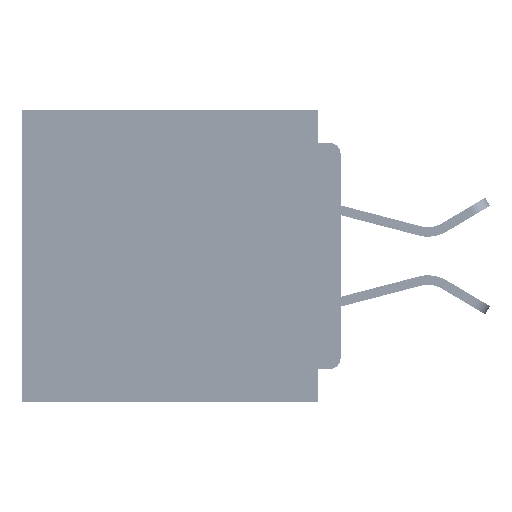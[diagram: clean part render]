
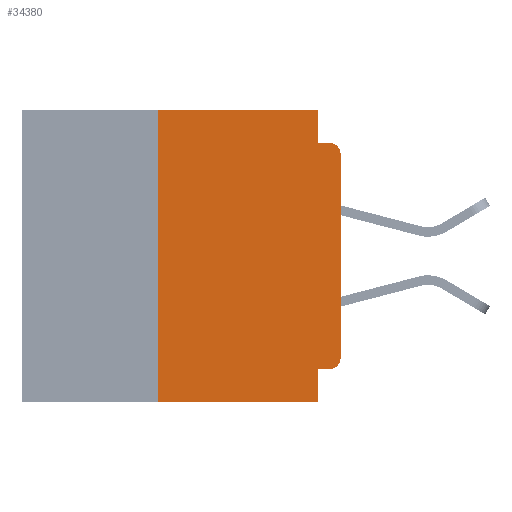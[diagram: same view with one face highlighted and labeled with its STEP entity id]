
A CAD part, left-side view. The second image highlights one B-rep face of the part: STEP entity #34380.
In plain terms, the highlighted planar face has unit normal (-1, 0, 0).
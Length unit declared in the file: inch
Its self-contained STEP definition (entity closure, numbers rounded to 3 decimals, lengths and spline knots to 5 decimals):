
#99 = VECTOR ( 'NONE', #842, 39.37008 ) ;
#659 = VECTOR ( 'NONE', #51162, 39.37008 ) ;
#842 = DIRECTION ( 'NONE',  ( 0., 0., -1. ) ) ;
#1524 = EDGE_CURVE ( 'NONE', #34058, #25634, #24173, .T. ) ;
#1538 = CARTESIAN_POINT ( 'NONE',  ( 0., 0., -0.34 ) ) ;
#2293 = VERTEX_POINT ( 'NONE', #41181 ) ;
#2834 = VECTOR ( 'NONE', #7046, 39.37008 ) ;
#2990 = CARTESIAN_POINT ( 'NONE',  ( 0., 0.031, -0.4 ) ) ;
#5468 = VECTOR ( 'NONE', #60756, 39.37008 ) ;
#6191 = CARTESIAN_POINT ( 'NONE',  ( 0., 0.015, -0.355 ) ) ;
#6379 = CARTESIAN_POINT ( 'NONE',  ( 0., 0.015, -0.34 ) ) ;
#7046 = DIRECTION ( 'NONE',  ( 0., -1., 0. ) ) ;
#7738 = VERTEX_POINT ( 'NONE', #44870 ) ;
#7950 = CARTESIAN_POINT ( 'NONE',  ( 0., 0.015, -0.045 ) ) ;
#8691 = DIRECTION ( 'NONE',  ( 0., 0., -1. ) ) ;
#9320 = EDGE_CURVE ( 'NONE', #7738, #52617, #40028, .T. ) ;
#9327 = AXIS2_PLACEMENT_3D ( 'NONE', #32891, #37742, #8691 ) ;
#9519 = AXIS2_PLACEMENT_3D ( 'NONE', #54440, #25648, #59216 ) ;
#9685 = AXIS2_PLACEMENT_3D ( 'NONE', #6379, #40273, #11241 ) ;
#10809 = DIRECTION ( 'NONE',  ( 0., -1., 0. ) ) ;
#11241 = DIRECTION ( 'NONE',  ( 0., 0., -1. ) ) ;
#11503 = EDGE_CURVE ( 'NONE', #52617, #2293, #13530, .T. ) ;
#11518 = CIRCLE ( 'NONE', #9685, 0.015 ) ;
#13530 = LINE ( 'NONE', #46327, #659 ) ;
#13780 = VECTOR ( 'NONE', #10809, 39.37008 ) ;
#15394 = EDGE_CURVE ( 'NONE', #29434, #55348, #33527, .T. ) ;
#15778 = VECTOR ( 'NONE', #33908, 39.37008 ) ;
#16578 = CARTESIAN_POINT ( 'NONE',  ( 0., 0., -0.045 ) ) ;
#16606 = CARTESIAN_POINT ( 'NONE',  ( 0., 0.25, -0.4 ) ) ;
#16900 = ORIENTED_EDGE ( 'NONE', *, *, #9320, .F. ) ;
#17994 = EDGE_LOOP ( 'NONE', ( #53447, #20706, #44732, #55438, #33008, #16900, #32135, #35148, #19680, #34286 ) ) ;
#18685 = CIRCLE ( 'NONE', #9519, 0.015 ) ;
#19680 = ORIENTED_EDGE ( 'NONE', *, *, #1524, .F. ) ;
#20377 = CARTESIAN_POINT ( 'NONE',  ( 0., 0.437, -0.4 ) ) ;
#20535 = FACE_OUTER_BOUND ( 'NONE', #17994, .T. ) ;
#20706 = ORIENTED_EDGE ( 'NONE', *, *, #41614, .T. ) ;
#21801 = CARTESIAN_POINT ( 'NONE',  ( 0., 0.031, -0.4 ) ) ;
#23041 = EDGE_CURVE ( 'NONE', #2293, #54435, #59716, .T. ) ;
#23720 = VECTOR ( 'NONE', #58821, 39.37008 ) ;
#24173 = LINE ( 'NONE', #54719, #48326 ) ;
#24492 = EDGE_CURVE ( 'NONE', #25634, #38003, #31297, .T. ) ;
#25039 = CARTESIAN_POINT ( 'NONE',  ( 0., 0.031, 0. ) ) ;
#25634 = VERTEX_POINT ( 'NONE', #30950 ) ;
#25648 = DIRECTION ( 'NONE',  ( -1., 0., 0. ) ) ;
#26277 = CARTESIAN_POINT ( 'NONE',  ( 0., 0.25, 0. ) ) ;
#29434 = VERTEX_POINT ( 'NONE', #1538 ) ;
#30107 = CARTESIAN_POINT ( 'NONE',  ( 0., 0., 0. ) ) ;
#30950 = CARTESIAN_POINT ( 'NONE',  ( 0., 0.031, -0.355 ) ) ;
#31297 = LINE ( 'NONE', #2990, #5468 ) ;
#32135 = ORIENTED_EDGE ( 'NONE', *, *, #51992, .T. ) ;
#32764 = VERTEX_POINT ( 'NONE', #7950 ) ;
#32891 = CARTESIAN_POINT ( 'NONE',  ( 0., 0.437, 0. ) ) ;
#33008 = ORIENTED_EDGE ( 'NONE', *, *, #11503, .F. ) ;
#33527 = LINE ( 'NONE', #30107, #23720 ) ;
#33690 = EDGE_CURVE ( 'NONE', #34058, #29434, #11518, .T. ) ;
#33908 = DIRECTION ( 'NONE',  ( 0., 0., 1. ) ) ;
#34058 = VERTEX_POINT ( 'NONE', #6191 ) ;
#34286 = ORIENTED_EDGE ( 'NONE', *, *, #33690, .T. ) ;
#34380 = ADVANCED_FACE ( 'NONE', ( #20535 ), #61557, .F. ) ;
#35148 = ORIENTED_EDGE ( 'NONE', *, *, #24492, .F. ) ;
#37742 = DIRECTION ( 'NONE',  ( 1., 0., 0. ) ) ;
#38003 = VERTEX_POINT ( 'NONE', #21801 ) ;
#40028 = LINE ( 'NONE', #16606, #15778 ) ;
#40273 = DIRECTION ( 'NONE',  ( -1., 0., 0. ) ) ;
#41181 = CARTESIAN_POINT ( 'NONE',  ( 0., 0.031, 0. ) ) ;
#41521 = LINE ( 'NONE', #16578, #2834 ) ;
#41614 = EDGE_CURVE ( 'NONE', #55348, #32764, #18685, .T. ) ;
#42900 = CARTESIAN_POINT ( 'NONE',  ( 0., 0.031, -0.045 ) ) ;
#44732 = ORIENTED_EDGE ( 'NONE', *, *, #59800, .F. ) ;
#44870 = CARTESIAN_POINT ( 'NONE',  ( 0., 0.25, -0.4 ) ) ;
#46327 = CARTESIAN_POINT ( 'NONE',  ( 0., 0.437, 0. ) ) ;
#48326 = VECTOR ( 'NONE', #55194, 39.37008 ) ;
#51162 = DIRECTION ( 'NONE',  ( 0., -1., 0. ) ) ;
#51992 = EDGE_CURVE ( 'NONE', #7738, #38003, #53804, .T. ) ;
#52617 = VERTEX_POINT ( 'NONE', #26277 ) ;
#53447 = ORIENTED_EDGE ( 'NONE', *, *, #15394, .T. ) ;
#53804 = LINE ( 'NONE', #20377, #13780 ) ;
#54435 = VERTEX_POINT ( 'NONE', #42900 ) ;
#54440 = CARTESIAN_POINT ( 'NONE',  ( 0., 0.015, -0.06 ) ) ;
#54719 = CARTESIAN_POINT ( 'NONE',  ( 0., 0., -0.355 ) ) ;
#55194 = DIRECTION ( 'NONE',  ( 0., 1., 0. ) ) ;
#55322 = CARTESIAN_POINT ( 'NONE',  ( 0., 0., -0.06 ) ) ;
#55348 = VERTEX_POINT ( 'NONE', #55322 ) ;
#55438 = ORIENTED_EDGE ( 'NONE', *, *, #23041, .F. ) ;
#58821 = DIRECTION ( 'NONE',  ( 0., 0., 1. ) ) ;
#59216 = DIRECTION ( 'NONE',  ( 0., 0., -1. ) ) ;
#59716 = LINE ( 'NONE', #25039, #99 ) ;
#59800 = EDGE_CURVE ( 'NONE', #54435, #32764, #41521, .T. ) ;
#60756 = DIRECTION ( 'NONE',  ( 0., 0., -1. ) ) ;
#61557 = PLANE ( 'NONE',  #9327 ) ;
